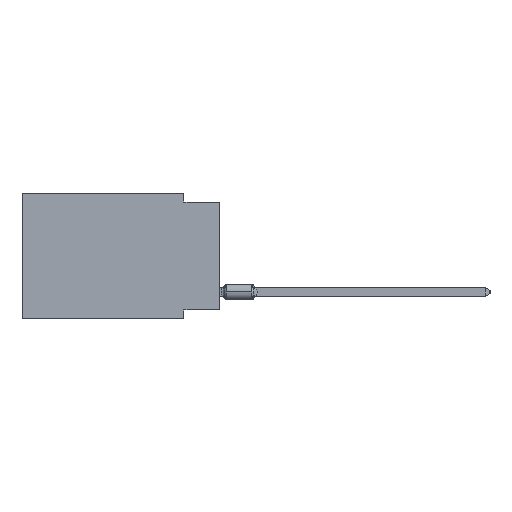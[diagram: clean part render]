
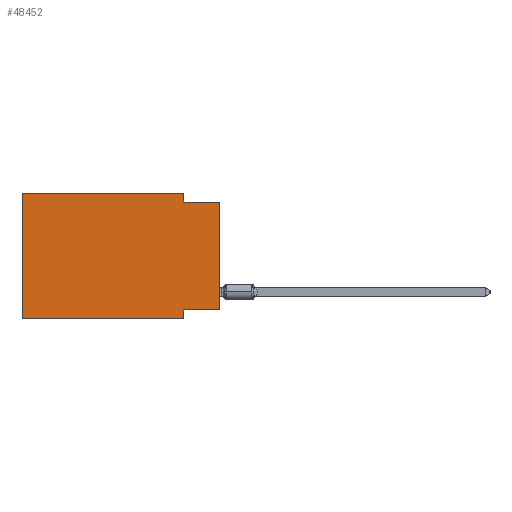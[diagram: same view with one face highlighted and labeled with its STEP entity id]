
A CAD part, left-side view. The second image highlights one B-rep face of the part: STEP entity #48452.
In plain terms, the highlighted planar face has unit normal (-1, 0, 0).
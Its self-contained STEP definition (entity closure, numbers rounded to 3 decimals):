
#2334 = VECTOR ( 'NONE', #51582, 1000. ) ;
#2407 = VECTOR ( 'NONE', #36440, 1000. ) ;
#3071 = ORIENTED_EDGE ( 'NONE', *, *, #15274, .T. ) ;
#3714 = ORIENTED_EDGE ( 'NONE', *, *, #6678, .F. ) ;
#4248 = VECTOR ( 'NONE', #5351, 1000. ) ;
#5351 = DIRECTION ( 'NONE',  ( 0., 0., -1. ) ) ;
#5689 = DIRECTION ( 'NONE',  ( 0., 0., 1. ) ) ;
#6288 = CARTESIAN_POINT ( 'NONE',  ( 0., 13.97, 0. ) ) ;
#6678 = EDGE_CURVE ( 'NONE', #53698, #26896, #54132, .T. ) ;
#8056 = VECTOR ( 'NONE', #38379, 1000. ) ;
#8269 = VERTEX_POINT ( 'NONE', #43770 ) ;
#8445 = EDGE_CURVE ( 'NONE', #26896, #8269, #53333, .T. ) ;
#9297 = AXIS2_PLACEMENT_3D ( 'NONE', #28239, #16095, #53861 ) ;
#12300 = ORIENTED_EDGE ( 'NONE', *, *, #8445, .F. ) ;
#13695 = CARTESIAN_POINT ( 'NONE',  ( 0., 0., -8.255 ) ) ;
#14808 = VERTEX_POINT ( 'NONE', #36043 ) ;
#15274 = EDGE_CURVE ( 'NONE', #53698, #14808, #32521, .T. ) ;
#15514 = ORIENTED_EDGE ( 'NONE', *, *, #39016, .T. ) ;
#16095 = DIRECTION ( 'NONE',  ( 1., 0., 0. ) ) ;
#16257 = CARTESIAN_POINT ( 'NONE',  ( 0., 2.54, -8.255 ) ) ;
#18075 = CARTESIAN_POINT ( 'NONE',  ( 0., 0., -0.635 ) ) ;
#20053 = DIRECTION ( 'NONE',  ( 0., 0., 1. ) ) ;
#20054 = CARTESIAN_POINT ( 'NONE',  ( 0., 0., -8.255 ) ) ;
#20614 = LINE ( 'NONE', #20054, #50028 ) ;
#20662 = CARTESIAN_POINT ( 'NONE',  ( 0., 13.97, -8.89 ) ) ;
#21833 = CARTESIAN_POINT ( 'NONE',  ( 0., 0., -0.635 ) ) ;
#22448 = EDGE_CURVE ( 'NONE', #31338, #14808, #48130, .T. ) ;
#23052 = CARTESIAN_POINT ( 'NONE',  ( 0., 13.97, 0. ) ) ;
#23064 = CARTESIAN_POINT ( 'NONE',  ( 0., 2.54, -0.635 ) ) ;
#25172 = VERTEX_POINT ( 'NONE', #23064 ) ;
#25422 = LINE ( 'NONE', #42865, #2334 ) ;
#25997 = ORIENTED_EDGE ( 'NONE', *, *, #22448, .F. ) ;
#26896 = VERTEX_POINT ( 'NONE', #23052 ) ;
#28239 = CARTESIAN_POINT ( 'NONE',  ( 0., 13.97, 0. ) ) ;
#30002 = DIRECTION ( 'NONE',  ( 0., -1., 0. ) ) ;
#30103 = ORIENTED_EDGE ( 'NONE', *, *, #52064, .F. ) ;
#30418 = VERTEX_POINT ( 'NONE', #13695 ) ;
#31338 = VERTEX_POINT ( 'NONE', #16257 ) ;
#32521 = LINE ( 'NONE', #20662, #8056 ) ;
#33370 = EDGE_CURVE ( 'NONE', #8269, #25172, #25422, .T. ) ;
#34793 = LINE ( 'NONE', #21833, #39386 ) ;
#35864 = ORIENTED_EDGE ( 'NONE', *, *, #33370, .F. ) ;
#36043 = CARTESIAN_POINT ( 'NONE',  ( 0., 2.54, -8.89 ) ) ;
#36440 = DIRECTION ( 'NONE',  ( 0., -1., 0. ) ) ;
#38379 = DIRECTION ( 'NONE',  ( 0., -1., 0. ) ) ;
#39016 = EDGE_CURVE ( 'NONE', #30418, #43389, #44261, .T. ) ;
#39386 = VECTOR ( 'NONE', #30002, 1000. ) ;
#39973 = CARTESIAN_POINT ( 'NONE',  ( 0., 2.54, -8.89 ) ) ;
#42239 = ORIENTED_EDGE ( 'NONE', *, *, #46575, .F. ) ;
#42865 = CARTESIAN_POINT ( 'NONE',  ( 0., 2.54, 0. ) ) ;
#43389 = VERTEX_POINT ( 'NONE', #18075 ) ;
#43770 = CARTESIAN_POINT ( 'NONE',  ( 0., 2.54, 0. ) ) ;
#43994 = CARTESIAN_POINT ( 'NONE',  ( 0., 0., 0. ) ) ;
#44261 = LINE ( 'NONE', #43994, #48881 ) ;
#44690 = CARTESIAN_POINT ( 'NONE',  ( 0., 13.97, -8.89 ) ) ;
#46495 = DIRECTION ( 'NONE',  ( 0., 1., 0. ) ) ;
#46575 = EDGE_CURVE ( 'NONE', #25172, #43389, #34793, .T. ) ;
#48130 = LINE ( 'NONE', #39973, #4248 ) ;
#48452 = ADVANCED_FACE ( 'NONE', ( #54393 ), #50700, .F. ) ;
#48881 = VECTOR ( 'NONE', #5689, 1000. ) ;
#49406 = EDGE_LOOP ( 'NONE', ( #15514, #42239, #35864, #12300, #3714, #3071, #25997, #30103 ) ) ;
#50028 = VECTOR ( 'NONE', #46495, 1000. ) ;
#50215 = CARTESIAN_POINT ( 'NONE',  ( 0., 13.97, 0. ) ) ;
#50700 = PLANE ( 'NONE',  #9297 ) ;
#51582 = DIRECTION ( 'NONE',  ( 0., 0., -1. ) ) ;
#51800 = VECTOR ( 'NONE', #20053, 1000. ) ;
#52064 = EDGE_CURVE ( 'NONE', #30418, #31338, #20614, .T. ) ;
#53333 = LINE ( 'NONE', #50215, #2407 ) ;
#53698 = VERTEX_POINT ( 'NONE', #44690 ) ;
#53861 = DIRECTION ( 'NONE',  ( 0., 0., -1. ) ) ;
#54132 = LINE ( 'NONE', #6288, #51800 ) ;
#54393 = FACE_OUTER_BOUND ( 'NONE', #49406, .T. ) ;
